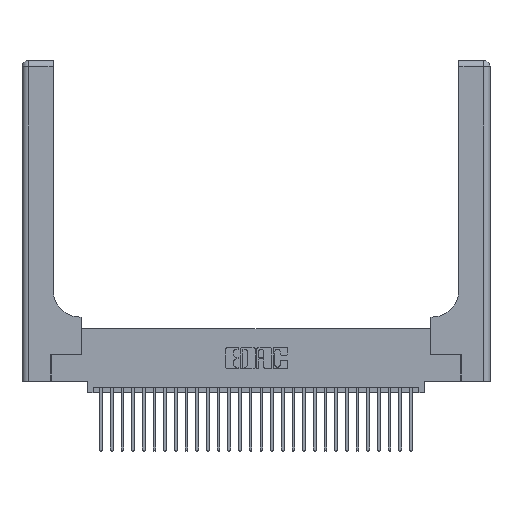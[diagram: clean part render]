
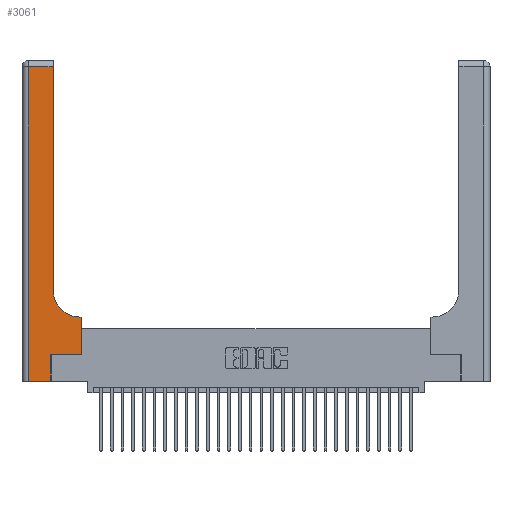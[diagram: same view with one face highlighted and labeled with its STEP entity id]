
A CAD part, top view. The second image highlights one B-rep face of the part: STEP entity #3061.
In plain terms, the highlighted planar face has unit normal (0, 0, 1).
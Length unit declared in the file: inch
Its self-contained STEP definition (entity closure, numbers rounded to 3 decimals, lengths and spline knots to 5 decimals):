
#785 = CARTESIAN_POINT ( 'NONE',  ( 0.2915, 0.6, 0.37 ) ) ;
#1051 = EDGE_CURVE ( 'NONE', #6284, #29169, #11177, .T. ) ;
#1246 = CARTESIAN_POINT ( 'NONE',  ( 0., 3., 0.37 ) ) ;
#1344 = ORIENTED_EDGE ( 'NONE', *, *, #1051, .T. ) ;
#1812 = ORIENTED_EDGE ( 'NONE', *, *, #15211, .T. ) ;
#3061 = ADVANCED_FACE ( 'NONE', ( #8840 ), #20246, .F. ) ;
#3417 = CARTESIAN_POINT ( 'NONE',  ( 0.269, 0.25, 0.37 ) ) ;
#3790 = ORIENTED_EDGE ( 'NONE', *, *, #3807, .T. ) ;
#3807 = EDGE_CURVE ( 'NONE', #21039, #19587, #25724, .T. ) ;
#4486 = VERTEX_POINT ( 'NONE', #23459 ) ;
#4868 = EDGE_CURVE ( 'NONE', #20682, #28909, #9898, .T. ) ;
#5319 = CARTESIAN_POINT ( 'NONE',  ( 0.5415, 0.6, 0.37 ) ) ;
#5730 = EDGE_LOOP ( 'NONE', ( #7686, #21302, #23298, #11076, #1812, #22043, #3790, #26703, #1344 ) ) ;
#5822 = CARTESIAN_POINT ( 'NONE',  ( 0.5415, 0.85, 0.37 ) ) ;
#6080 = DIRECTION ( 'NONE',  ( 0., -1., 0. ) ) ;
#6135 = DIRECTION ( 'NONE',  ( 0., 0., -1. ) ) ;
#6284 = VERTEX_POINT ( 'NONE', #5319 ) ;
#6594 = CARTESIAN_POINT ( 'NONE',  ( 0.5585, 0.25, 0.37 ) ) ;
#6842 = LINE ( 'NONE', #27755, #12405 ) ;
#6966 = EDGE_CURVE ( 'NONE', #19587, #6284, #14162, .T. ) ;
#7225 = DIRECTION ( 'NONE',  ( 0., 1., 0. ) ) ;
#7686 = ORIENTED_EDGE ( 'NONE', *, *, #12239, .T. ) ;
#7939 = DIRECTION ( 'NONE',  ( -1., 0., 0. ) ) ;
#8184 = DIRECTION ( 'NONE',  ( 1., 0., 0. ) ) ;
#8618 = CARTESIAN_POINT ( 'NONE',  ( 0.5585, 0.6, 0.37 ) ) ;
#8840 = FACE_OUTER_BOUND ( 'NONE', #5730, .T. ) ;
#8843 = EDGE_CURVE ( 'NONE', #25041, #21039, #16629, .T. ) ;
#8855 = CARTESIAN_POINT ( 'NONE',  ( 0.06, 3., 0.37 ) ) ;
#8953 = DIRECTION ( 'NONE',  ( 0., 1., 0. ) ) ;
#9142 = VECTOR ( 'NONE', #22405, 39.37008 ) ;
#9187 = CARTESIAN_POINT ( 'NONE',  ( 0.2915, 0.85, 0.37 ) ) ;
#9681 = CARTESIAN_POINT ( 'NONE',  ( 0.5585, 0.25, 0.37 ) ) ;
#9898 = LINE ( 'NONE', #15325, #9142 ) ;
#10784 = CARTESIAN_POINT ( 'NONE',  ( 0.269, 0., 0.37 ) ) ;
#11076 = ORIENTED_EDGE ( 'NONE', *, *, #24887, .T. ) ;
#11177 = CIRCLE ( 'NONE', #28828, 0.25 ) ;
#12239 = EDGE_CURVE ( 'NONE', #29169, #20682, #22688, .T. ) ;
#12405 = VECTOR ( 'NONE', #16091, 39.37008 ) ;
#14162 = LINE ( 'NONE', #785, #19678 ) ;
#15211 = EDGE_CURVE ( 'NONE', #15734, #25041, #6842, .T. ) ;
#15325 = CARTESIAN_POINT ( 'NONE',  ( 0., 2.94, 0.37 ) ) ;
#15734 = VERTEX_POINT ( 'NONE', #10784 ) ;
#16091 = DIRECTION ( 'NONE',  ( 0., 1., 0. ) ) ;
#16629 = LINE ( 'NONE', #3417, #28331 ) ;
#16790 = CARTESIAN_POINT ( 'NONE',  ( 0.06, 2.94, 0.37 ) ) ;
#17211 = VECTOR ( 'NONE', #7225, 39.37008 ) ;
#17656 = DIRECTION ( 'NONE',  ( 1., 0., 0. ) ) ;
#18677 = DIRECTION ( 'NONE',  ( 1., 0., 0. ) ) ;
#19587 = VERTEX_POINT ( 'NONE', #8618 ) ;
#19678 = VECTOR ( 'NONE', #7939, 39.37008 ) ;
#20246 = PLANE ( 'NONE',  #23770 ) ;
#20682 = VERTEX_POINT ( 'NONE', #25022 ) ;
#21039 = VERTEX_POINT ( 'NONE', #9681 ) ;
#21302 = ORIENTED_EDGE ( 'NONE', *, *, #4868, .T. ) ;
#21307 = CARTESIAN_POINT ( 'NONE',  ( 0.2915, 3., 0.37 ) ) ;
#22043 = ORIENTED_EDGE ( 'NONE', *, *, #8843, .T. ) ;
#22299 = DIRECTION ( 'NONE',  ( 0., 0., -1. ) ) ;
#22405 = DIRECTION ( 'NONE',  ( -1., 0., 0. ) ) ;
#22604 = DIRECTION ( 'NONE',  ( -1., 0., 0. ) ) ;
#22688 = LINE ( 'NONE', #21307, #17211 ) ;
#23298 = ORIENTED_EDGE ( 'NONE', *, *, #25355, .T. ) ;
#23406 = CARTESIAN_POINT ( 'NONE',  ( 0., 0., 0.37 ) ) ;
#23459 = CARTESIAN_POINT ( 'NONE',  ( 0.06, 0., 0.37 ) ) ;
#23770 = AXIS2_PLACEMENT_3D ( 'NONE', #1246, #6135, #22604 ) ;
#24434 = VECTOR ( 'NONE', #6080, 39.37008 ) ;
#24887 = EDGE_CURVE ( 'NONE', #4486, #15734, #29200, .T. ) ;
#25003 = VECTOR ( 'NONE', #8953, 39.37008 ) ;
#25022 = CARTESIAN_POINT ( 'NONE',  ( 0.2915, 2.94, 0.37 ) ) ;
#25041 = VERTEX_POINT ( 'NONE', #26129 ) ;
#25355 = EDGE_CURVE ( 'NONE', #28909, #4486, #29894, .T. ) ;
#25724 = LINE ( 'NONE', #6594, #25003 ) ;
#26129 = CARTESIAN_POINT ( 'NONE',  ( 0.269, 0.25, 0.37 ) ) ;
#26703 = ORIENTED_EDGE ( 'NONE', *, *, #6966, .T. ) ;
#27755 = CARTESIAN_POINT ( 'NONE',  ( 0.269, 0., 0.37 ) ) ;
#28331 = VECTOR ( 'NONE', #17656, 39.37008 ) ;
#28828 = AXIS2_PLACEMENT_3D ( 'NONE', #5822, #22299, #8184 ) ;
#28909 = VERTEX_POINT ( 'NONE', #16790 ) ;
#29169 = VERTEX_POINT ( 'NONE', #9187 ) ;
#29200 = LINE ( 'NONE', #23406, #29924 ) ;
#29894 = LINE ( 'NONE', #8855, #24434 ) ;
#29924 = VECTOR ( 'NONE', #18677, 39.37008 ) ;
